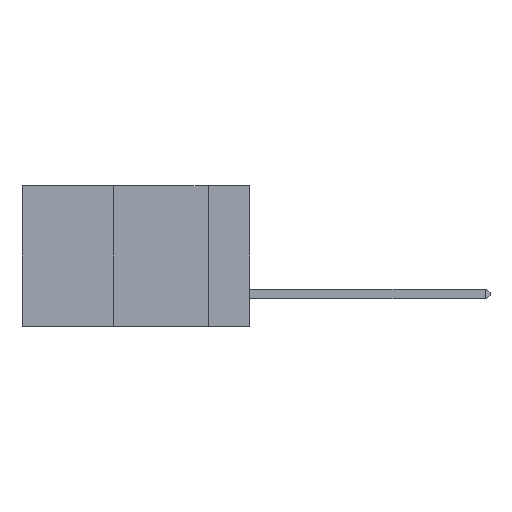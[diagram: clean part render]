
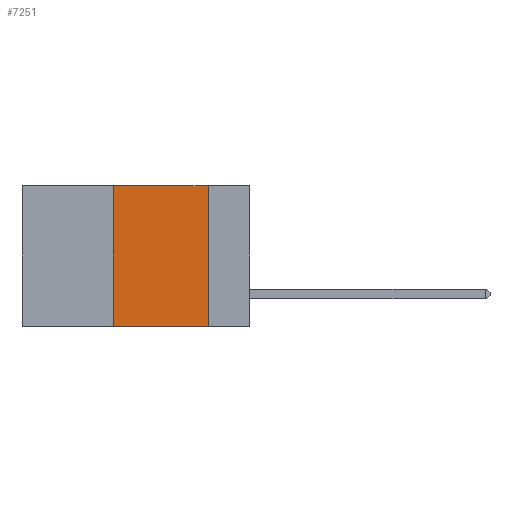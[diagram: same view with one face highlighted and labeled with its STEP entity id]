
A CAD part, left-side view. The second image highlights one B-rep face of the part: STEP entity #7251.
In plain terms, the highlighted planar face has unit normal (-1, 0, 0).
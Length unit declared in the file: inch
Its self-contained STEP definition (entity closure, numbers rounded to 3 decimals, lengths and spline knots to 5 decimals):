
#360 = PLANE ( 'NONE',  #12506 ) ;
#407 = EDGE_CURVE ( 'NONE', #5733, #14997, #14329, .T. ) ;
#951 = LINE ( 'NONE', #4990, #7464 ) ;
#986 = CARTESIAN_POINT ( 'NONE',  ( 0., 0.11, 0. ) ) ;
#1739 = CARTESIAN_POINT ( 'NONE',  ( 0., 0.6, 0. ) ) ;
#2463 = CARTESIAN_POINT ( 'NONE',  ( 0., 0.11, 0. ) ) ;
#3116 = DIRECTION ( 'NONE',  ( 0., 0., -1. ) ) ;
#3242 = FACE_OUTER_BOUND ( 'NONE', #13093, .T. ) ;
#4352 = ORIENTED_EDGE ( 'NONE', *, *, #14088, .F. ) ;
#4990 = CARTESIAN_POINT ( 'NONE',  ( 0., 0.6, 0. ) ) ;
#5267 = VECTOR ( 'NONE', #15249, 39.37008 ) ;
#5676 = CARTESIAN_POINT ( 'NONE',  ( 0., 0.11, -0.37 ) ) ;
#5733 = VERTEX_POINT ( 'NONE', #12858 ) ;
#5917 = CARTESIAN_POINT ( 'NONE',  ( 0., 0.36, 0. ) ) ;
#6375 = VECTOR ( 'NONE', #9935, 39.37008 ) ;
#6738 = CARTESIAN_POINT ( 'NONE',  ( 0., 0.6, -0.37 ) ) ;
#6811 = CARTESIAN_POINT ( 'NONE',  ( 0., 0.36, 0. ) ) ;
#6829 = DIRECTION ( 'NONE',  ( 0., 0., 1. ) ) ;
#7164 = EDGE_CURVE ( 'NONE', #5733, #12633, #11353, .T. ) ;
#7251 = ADVANCED_FACE ( 'NONE', ( #3242 ), #360, .F. ) ;
#7464 = VECTOR ( 'NONE', #7520, 39.37008 ) ;
#7520 = DIRECTION ( 'NONE',  ( 0., -1., 0. ) ) ;
#9291 = VERTEX_POINT ( 'NONE', #986 ) ;
#9309 = EDGE_CURVE ( 'NONE', #14997, #9291, #951, .T. ) ;
#9568 = LINE ( 'NONE', #2463, #6375 ) ;
#9935 = DIRECTION ( 'NONE',  ( 0., 0., -1. ) ) ;
#10498 = DIRECTION ( 'NONE',  ( 1., 0., 0. ) ) ;
#11046 = VECTOR ( 'NONE', #6829, 39.37008 ) ;
#11230 = ORIENTED_EDGE ( 'NONE', *, *, #407, .F. ) ;
#11353 = LINE ( 'NONE', #6738, #5267 ) ;
#12506 = AXIS2_PLACEMENT_3D ( 'NONE', #1739, #10498, #3116 ) ;
#12633 = VERTEX_POINT ( 'NONE', #5676 ) ;
#12858 = CARTESIAN_POINT ( 'NONE',  ( 0., 0.36, -0.37 ) ) ;
#13093 = EDGE_LOOP ( 'NONE', ( #4352, #14118, #11230, #14897 ) ) ;
#14088 = EDGE_CURVE ( 'NONE', #9291, #12633, #9568, .T. ) ;
#14118 = ORIENTED_EDGE ( 'NONE', *, *, #9309, .F. ) ;
#14329 = LINE ( 'NONE', #6811, #11046 ) ;
#14897 = ORIENTED_EDGE ( 'NONE', *, *, #7164, .T. ) ;
#14997 = VERTEX_POINT ( 'NONE', #5917 ) ;
#15249 = DIRECTION ( 'NONE',  ( 0., -1., 0. ) ) ;
